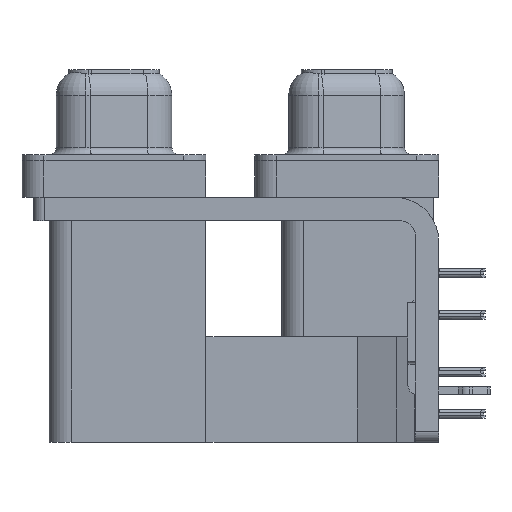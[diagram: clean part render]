
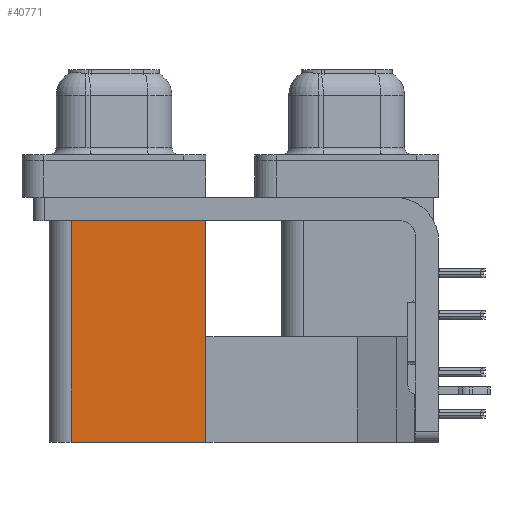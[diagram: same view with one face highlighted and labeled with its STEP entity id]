
A CAD part, left-side view. The second image highlights one B-rep face of the part: STEP entity #40771.
In plain terms, the highlighted planar face has unit normal (-1, 0, 0).
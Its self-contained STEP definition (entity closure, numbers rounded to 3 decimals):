
#52 = LINE ( 'NONE', #37357, #15657 ) ;
#2092 = EDGE_CURVE ( 'NONE', #34050, #43770, #52, .T. ) ;
#3625 = CARTESIAN_POINT ( 'NONE',  ( 3.79, 9.6, -19.2 ) ) ;
#3920 = CARTESIAN_POINT ( 'NONE',  ( 3.79, 18.8, -19.2 ) ) ;
#4128 = CARTESIAN_POINT ( 'NONE',  ( 3.79, 9.6, -19.2 ) ) ;
#4927 = DIRECTION ( 'NONE',  ( 0., 0., 1. ) ) ;
#5145 = LINE ( 'NONE', #25172, #22121 ) ;
#6779 = VECTOR ( 'NONE', #17564, 1000. ) ;
#7148 = EDGE_CURVE ( 'NONE', #21724, #11298, #43775, .T. ) ;
#9833 = DIRECTION ( 'NONE',  ( 0., 1., 0. ) ) ;
#10230 = CARTESIAN_POINT ( 'NONE',  ( 3.79, 9.6, -2.5 ) ) ;
#10787 = DIRECTION ( 'NONE',  ( 0., 1., 0. ) ) ;
#11298 = VERTEX_POINT ( 'NONE', #27674 ) ;
#11609 = EDGE_CURVE ( 'NONE', #34050, #21724, #5145, .T. ) ;
#15657 = VECTOR ( 'NONE', #9833, 1000. ) ;
#17564 = DIRECTION ( 'NONE',  ( 0., 1., 0. ) ) ;
#18337 = ORIENTED_EDGE ( 'NONE', *, *, #26233, .F. ) ;
#19693 = CARTESIAN_POINT ( 'NONE',  ( 3.79, 9.6, -2.5 ) ) ;
#21724 = VERTEX_POINT ( 'NONE', #19693 ) ;
#22121 = VECTOR ( 'NONE', #4927, 1000. ) ;
#23721 = LINE ( 'NONE', #3920, #32497 ) ;
#24062 = ORIENTED_EDGE ( 'NONE', *, *, #11609, .T. ) ;
#24812 = ORIENTED_EDGE ( 'NONE', *, *, #2092, .F. ) ;
#25172 = CARTESIAN_POINT ( 'NONE',  ( 3.79, 9.6, -19.2 ) ) ;
#26233 = EDGE_CURVE ( 'NONE', #43770, #11298, #23721, .T. ) ;
#27674 = CARTESIAN_POINT ( 'NONE',  ( 3.79, 18.8, -2.5 ) ) ;
#27689 = FACE_OUTER_BOUND ( 'NONE', #38753, .T. ) ;
#28679 = AXIS2_PLACEMENT_3D ( 'NONE', #4128, #38101, #10787 ) ;
#31312 = CARTESIAN_POINT ( 'NONE',  ( 3.79, 18.8, -19.2 ) ) ;
#32497 = VECTOR ( 'NONE', #34121, 1000. ) ;
#34050 = VERTEX_POINT ( 'NONE', #3625 ) ;
#34121 = DIRECTION ( 'NONE',  ( 0., 0., 1. ) ) ;
#37357 = CARTESIAN_POINT ( 'NONE',  ( 3.79, 9.6, -19.2 ) ) ;
#38101 = DIRECTION ( 'NONE',  ( 1., 0., 0. ) ) ;
#38753 = EDGE_LOOP ( 'NONE', ( #41108, #18337, #24812, #24062 ) ) ;
#40771 = ADVANCED_FACE ( 'NONE', ( #27689 ), #41438, .F. ) ;
#41108 = ORIENTED_EDGE ( 'NONE', *, *, #7148, .T. ) ;
#41438 = PLANE ( 'NONE',  #28679 ) ;
#43770 = VERTEX_POINT ( 'NONE', #31312 ) ;
#43775 = LINE ( 'NONE', #10230, #6779 ) ;
